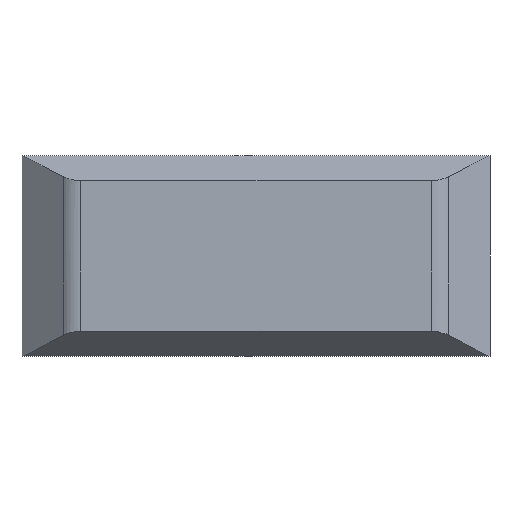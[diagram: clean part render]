
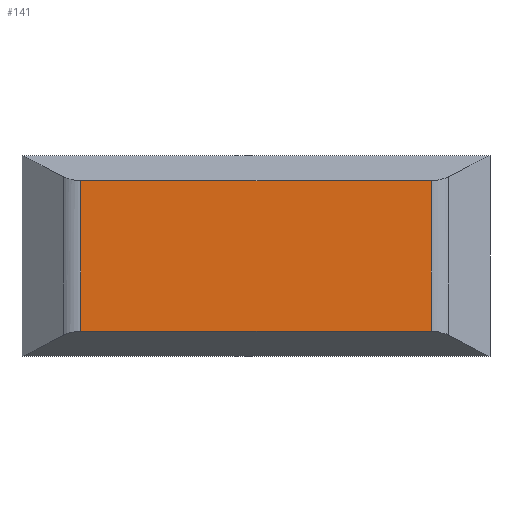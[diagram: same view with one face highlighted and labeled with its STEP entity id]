
A CAD part, top view. The second image highlights one B-rep face of the part: STEP entity #141.
In plain terms, the highlighted planar face has unit normal (0, 0, 1).
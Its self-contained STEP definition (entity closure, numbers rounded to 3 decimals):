
#21=FACE_OUTER_BOUND('',#29,.T.);
#29=EDGE_LOOP('',(#115,#116,#117,#118));
#40=LINE('',#223,#54);
#42=LINE('',#232,#56);
#47=LINE('',#242,#61);
#48=LINE('',#244,#62);
#54=VECTOR('',#180,10.);
#56=VECTOR('',#188,10.);
#61=VECTOR('',#199,10.);
#62=VECTOR('',#202,10.);
#69=VERTEX_POINT('',#220);
#70=VERTEX_POINT('',#222);
#73=VERTEX_POINT('',#229);
#74=VERTEX_POINT('',#231);
#81=EDGE_CURVE('',#70,#69,#40,.T.);
#85=EDGE_CURVE('',#74,#73,#42,.T.);
#91=EDGE_CURVE('',#70,#73,#47,.T.);
#92=EDGE_CURVE('',#74,#69,#48,.T.);
#115=ORIENTED_EDGE('',*,*,#81,.T.);
#116=ORIENTED_EDGE('',*,*,#92,.F.);
#117=ORIENTED_EDGE('',*,*,#85,.T.);
#118=ORIENTED_EDGE('',*,*,#91,.F.);
#134=PLANE('',#167);
#141=ADVANCED_FACE('',(#21),#134,.T.);
#167=AXIS2_PLACEMENT_3D('',#243,#200,#201);
#180=DIRECTION('',(1.,0.,0.));
#188=DIRECTION('',(-1.,0.,0.));
#199=DIRECTION('',(0.,1.,0.));
#200=DIRECTION('center_axis',(0.,0.,1.));
#201=DIRECTION('ref_axis',(1.,0.,0.));
#202=DIRECTION('',(0.,-1.,0.));
#220=CARTESIAN_POINT('',(15.478,0.95,1.6));
#222=CARTESIAN_POINT('',(2.222,0.95,1.6));
#223=CARTESIAN_POINT('',(13.275,0.95,1.6));
#229=CARTESIAN_POINT('',(2.222,6.65,1.6));
#231=CARTESIAN_POINT('',(15.478,6.65,1.6));
#232=CARTESIAN_POINT('',(13.275,6.65,1.6));
#242=CARTESIAN_POINT('',(2.222,1.9,1.6));
#243=CARTESIAN_POINT('Origin',(8.85,3.8,1.6));
#244=CARTESIAN_POINT('',(15.478,1.9,1.6));
